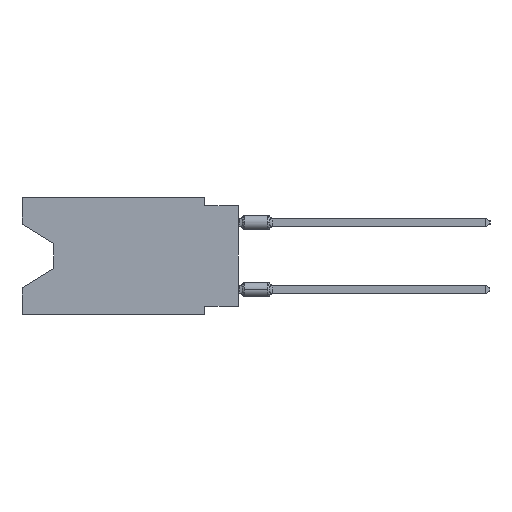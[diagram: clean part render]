
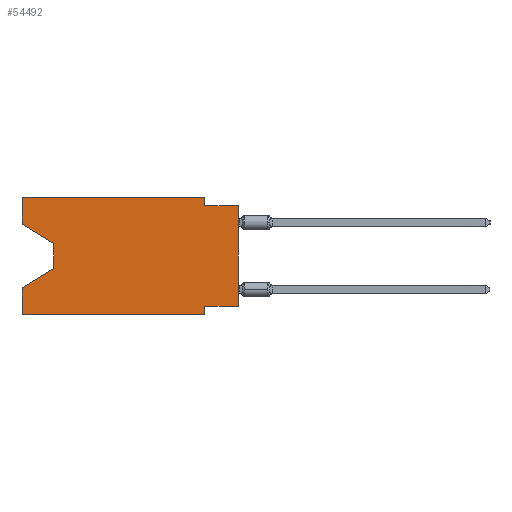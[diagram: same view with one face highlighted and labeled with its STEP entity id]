
A CAD part, left-side view. The second image highlights one B-rep face of the part: STEP entity #54492.
In plain terms, the highlighted planar face has unit normal (-1, 0, 0).
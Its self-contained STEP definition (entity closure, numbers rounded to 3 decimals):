
#2013 = LINE ( 'NONE', #25766, #47356 ) ;
#2234 = EDGE_CURVE ( 'NONE', #41319, #23045, #30410, .T. ) ;
#3069 = EDGE_CURVE ( 'NONE', #52101, #10889, #18357, .T. ) ;
#3100 = DIRECTION ( 'NONE',  ( 0., 0., -1. ) ) ;
#3178 = EDGE_CURVE ( 'NONE', #38705, #33939, #33306, .T. ) ;
#4025 = ORIENTED_EDGE ( 'NONE', *, *, #31554, .T. ) ;
#4177 = EDGE_CURVE ( 'NONE', #10886, #20821, #43846, .T. ) ;
#4726 = CARTESIAN_POINT ( 'NONE',  ( 0., 16.383, 0. ) ) ;
#6215 = EDGE_CURVE ( 'NONE', #44837, #10889, #15433, .T. ) ;
#6735 = ORIENTED_EDGE ( 'NONE', *, *, #26961, .F. ) ;
#7475 = VECTOR ( 'NONE', #53774, 1000. ) ;
#8308 = LINE ( 'NONE', #62853, #10289 ) ;
#10289 = VECTOR ( 'NONE', #18381, 1000. ) ;
#10886 = VERTEX_POINT ( 'NONE', #13952 ) ;
#10889 = VERTEX_POINT ( 'NONE', #44484 ) ;
#11725 = VECTOR ( 'NONE', #39311, 1000. ) ;
#12271 = CARTESIAN_POINT ( 'NONE',  ( 0., 0., -8.255 ) ) ;
#13952 = CARTESIAN_POINT ( 'NONE',  ( 0., 13.97, -5.385 ) ) ;
#14314 = CARTESIAN_POINT ( 'NONE',  ( 0., 2.54, 0. ) ) ;
#14562 = ORIENTED_EDGE ( 'NONE', *, *, #3178, .F. ) ;
#14750 = CARTESIAN_POINT ( 'NONE',  ( 0., 16.383, -8.89 ) ) ;
#14962 = LINE ( 'NONE', #20140, #22502 ) ;
#15319 = ORIENTED_EDGE ( 'NONE', *, *, #22615, .F. ) ;
#15433 = LINE ( 'NONE', #35242, #53493 ) ;
#15872 = VERTEX_POINT ( 'NONE', #21443 ) ;
#16376 = EDGE_CURVE ( 'NONE', #52101, #38705, #56768, .T. ) ;
#16419 = CARTESIAN_POINT ( 'NONE',  ( 0., 16.383, 0. ) ) ;
#16481 = CARTESIAN_POINT ( 'NONE',  ( 0., 13.97, -3.505 ) ) ;
#17028 = LINE ( 'NONE', #16419, #55223 ) ;
#17188 = VERTEX_POINT ( 'NONE', #14750 ) ;
#17705 = CARTESIAN_POINT ( 'NONE',  ( 0., 0., 0. ) ) ;
#18137 = CARTESIAN_POINT ( 'NONE',  ( 0., 16.383, 0. ) ) ;
#18357 = LINE ( 'NONE', #17705, #7475 ) ;
#18381 = DIRECTION ( 'NONE',  ( 0., 0., 1. ) ) ;
#20140 = CARTESIAN_POINT ( 'NONE',  ( 0., 13.97, -3.505 ) ) ;
#20757 = CARTESIAN_POINT ( 'NONE',  ( 0., 2.54, -0.635 ) ) ;
#20821 = VERTEX_POINT ( 'NONE', #32786 ) ;
#21038 = DIRECTION ( 'NONE',  ( 0., 1., 0. ) ) ;
#21322 = EDGE_LOOP ( 'NONE', ( #47257, #4025, #47641, #6735, #36532, #14562, #24557, #35747, #24774, #46293, #15319, #50292 ) ) ;
#21443 = CARTESIAN_POINT ( 'NONE',  ( 0., 2.54, 0. ) ) ;
#22296 = EDGE_CURVE ( 'NONE', #17188, #33939, #51559, .T. ) ;
#22502 = VECTOR ( 'NONE', #54597, 1000. ) ;
#22615 = EDGE_CURVE ( 'NONE', #26310, #15872, #17028, .T. ) ;
#23045 = VERTEX_POINT ( 'NONE', #16481 ) ;
#23389 = LINE ( 'NONE', #14314, #30205 ) ;
#24557 = ORIENTED_EDGE ( 'NONE', *, *, #16376, .F. ) ;
#24774 = ORIENTED_EDGE ( 'NONE', *, *, #6215, .F. ) ;
#25541 = DIRECTION ( 'NONE',  ( 0., -0.855, -0.519 ) ) ;
#25766 = CARTESIAN_POINT ( 'NONE',  ( 0., 16.383, 0. ) ) ;
#26310 = VERTEX_POINT ( 'NONE', #18137 ) ;
#26961 = EDGE_CURVE ( 'NONE', #17188, #20821, #8308, .T. ) ;
#30205 = VECTOR ( 'NONE', #47428, 1000. ) ;
#30410 = LINE ( 'NONE', #35919, #32340 ) ;
#30696 = CARTESIAN_POINT ( 'NONE',  ( 0., 2.54, -8.255 ) ) ;
#31554 = EDGE_CURVE ( 'NONE', #23045, #10886, #14962, .T. ) ;
#32340 = VECTOR ( 'NONE', #25541, 1000. ) ;
#32786 = CARTESIAN_POINT ( 'NONE',  ( 0., 16.383, -6.852 ) ) ;
#33152 = CARTESIAN_POINT ( 'NONE',  ( 0., 16.383, -2.038 ) ) ;
#33306 = LINE ( 'NONE', #58615, #41766 ) ;
#33939 = VERTEX_POINT ( 'NONE', #54189 ) ;
#34453 = CARTESIAN_POINT ( 'NONE',  ( 0., 13.97, -5.385 ) ) ;
#35242 = CARTESIAN_POINT ( 'NONE',  ( 0., 0., -0.635 ) ) ;
#35747 = ORIENTED_EDGE ( 'NONE', *, *, #3069, .T. ) ;
#35919 = CARTESIAN_POINT ( 'NONE',  ( 0., 16.383, -2.038 ) ) ;
#36532 = ORIENTED_EDGE ( 'NONE', *, *, #22296, .T. ) ;
#36538 = DIRECTION ( 'NONE',  ( 0., -1., 0. ) ) ;
#36931 = CARTESIAN_POINT ( 'NONE',  ( 0., 16.383, -8.89 ) ) ;
#38705 = VERTEX_POINT ( 'NONE', #30696 ) ;
#38808 = PLANE ( 'NONE',  #41870 ) ;
#39311 = DIRECTION ( 'NONE',  ( 0., 0.855, -0.519 ) ) ;
#41319 = VERTEX_POINT ( 'NONE', #33152 ) ;
#41363 = EDGE_CURVE ( 'NONE', #15872, #44837, #23389, .T. ) ;
#41766 = VECTOR ( 'NONE', #3100, 1000. ) ;
#41870 = AXIS2_PLACEMENT_3D ( 'NONE', #4726, #44667, #49557 ) ;
#43846 = LINE ( 'NONE', #34453, #11725 ) ;
#44484 = CARTESIAN_POINT ( 'NONE',  ( 0., 0., -0.635 ) ) ;
#44667 = DIRECTION ( 'NONE',  ( 1., 0., 0. ) ) ;
#44837 = VERTEX_POINT ( 'NONE', #20757 ) ;
#46293 = ORIENTED_EDGE ( 'NONE', *, *, #41363, .F. ) ;
#47257 = ORIENTED_EDGE ( 'NONE', *, *, #2234, .T. ) ;
#47356 = VECTOR ( 'NONE', #55953, 1000. ) ;
#47428 = DIRECTION ( 'NONE',  ( 0., 0., -1. ) ) ;
#47641 = ORIENTED_EDGE ( 'NONE', *, *, #4177, .T. ) ;
#49213 = FACE_OUTER_BOUND ( 'NONE', #21322, .T. ) ;
#49544 = VECTOR ( 'NONE', #21038, 1000. ) ;
#49557 = DIRECTION ( 'NONE',  ( 0., 0., -1. ) ) ;
#50292 = ORIENTED_EDGE ( 'NONE', *, *, #51186, .F. ) ;
#51186 = EDGE_CURVE ( 'NONE', #41319, #26310, #2013, .T. ) ;
#51559 = LINE ( 'NONE', #36931, #52069 ) ;
#52069 = VECTOR ( 'NONE', #56750, 1000. ) ;
#52101 = VERTEX_POINT ( 'NONE', #62161 ) ;
#53493 = VECTOR ( 'NONE', #63479, 1000. ) ;
#53774 = DIRECTION ( 'NONE',  ( 0., 0., 1. ) ) ;
#54189 = CARTESIAN_POINT ( 'NONE',  ( 0., 2.54, -8.89 ) ) ;
#54492 = ADVANCED_FACE ( 'NONE', ( #49213 ), #38808, .F. ) ;
#54597 = DIRECTION ( 'NONE',  ( 0., 0., -1. ) ) ;
#55223 = VECTOR ( 'NONE', #36538, 1000. ) ;
#55953 = DIRECTION ( 'NONE',  ( 0., 0., 1. ) ) ;
#56750 = DIRECTION ( 'NONE',  ( 0., -1., 0. ) ) ;
#56768 = LINE ( 'NONE', #12271, #49544 ) ;
#58615 = CARTESIAN_POINT ( 'NONE',  ( 0., 2.54, -8.89 ) ) ;
#62161 = CARTESIAN_POINT ( 'NONE',  ( 0., 0., -8.255 ) ) ;
#62853 = CARTESIAN_POINT ( 'NONE',  ( 0., 16.383, 0. ) ) ;
#63479 = DIRECTION ( 'NONE',  ( 0., -1., 0. ) ) ;
